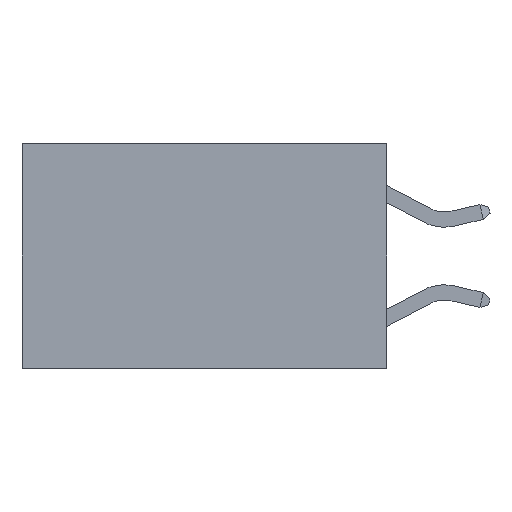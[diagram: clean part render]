
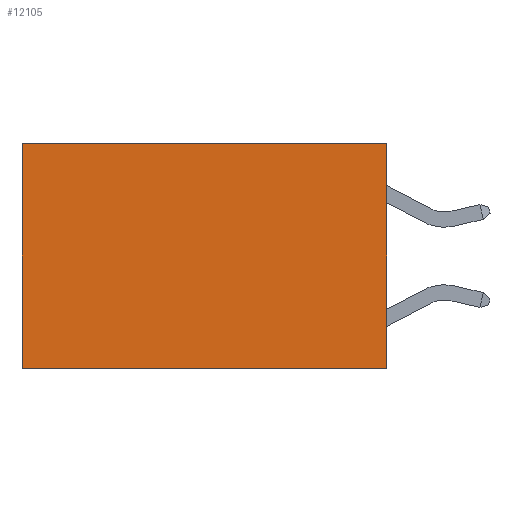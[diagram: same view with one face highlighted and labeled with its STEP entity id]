
A CAD part, left-side view. The second image highlights one B-rep face of the part: STEP entity #12105.
In plain terms, the highlighted planar face has unit normal (-1, 0, 0).
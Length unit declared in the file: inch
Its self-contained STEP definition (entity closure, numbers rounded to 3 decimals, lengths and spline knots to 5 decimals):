
#593 = DIRECTION ( 'NONE',  ( 0., 1., 0. ) ) ;
#1850 = VERTEX_POINT ( 'NONE', #5355 ) ;
#2541 = DIRECTION ( 'NONE',  ( 0., 1., 0. ) ) ;
#3790 = VECTOR ( 'NONE', #593, 39.37008 ) ;
#4301 = CARTESIAN_POINT ( 'NONE',  ( 0.2625, 0., 0. ) ) ;
#4383 = LINE ( 'NONE', #5997, #3790 ) ;
#4386 = DIRECTION ( 'NONE',  ( 0., 0., -1. ) ) ;
#4781 = AXIS2_PLACEMENT_3D ( 'NONE', #4301, #15117, #4386 ) ;
#5355 = CARTESIAN_POINT ( 'NONE',  ( 0.2625, 0., 0. ) ) ;
#5995 = VECTOR ( 'NONE', #2541, 39.37008 ) ;
#5997 = CARTESIAN_POINT ( 'NONE',  ( 0.2625, 0., -0.37 ) ) ;
#6035 = DIRECTION ( 'NONE',  ( 0., 0., -1. ) ) ;
#6043 = VECTOR ( 'NONE', #6035, 39.37008 ) ;
#6284 = LINE ( 'NONE', #15484, #19985 ) ;
#7701 = EDGE_CURVE ( 'NONE', #8911, #21904, #4383, .T. ) ;
#7807 = CARTESIAN_POINT ( 'NONE',  ( 0.2625, 0.6, 0. ) ) ;
#8381 = CARTESIAN_POINT ( 'NONE',  ( 0.2625, 0.6, 0. ) ) ;
#8502 = DIRECTION ( 'NONE',  ( 0., 0., -1. ) ) ;
#8504 = EDGE_CURVE ( 'NONE', #11580, #21904, #10812, .T. ) ;
#8738 = ORIENTED_EDGE ( 'NONE', *, *, #7701, .F. ) ;
#8911 = VERTEX_POINT ( 'NONE', #12494 ) ;
#10050 = EDGE_LOOP ( 'NONE', ( #18749, #8738, #15216, #20213 ) ) ;
#10812 = LINE ( 'NONE', #7807, #6043 ) ;
#11580 = VERTEX_POINT ( 'NONE', #8381 ) ;
#12105 = ADVANCED_FACE ( 'NONE', ( #21816 ), #22216, .F. ) ;
#12494 = CARTESIAN_POINT ( 'NONE',  ( 0.2625, 0., -0.37 ) ) ;
#13863 = CARTESIAN_POINT ( 'NONE',  ( 0.2625, 0.6, -0.37 ) ) ;
#15117 = DIRECTION ( 'NONE',  ( 1., 0., 0. ) ) ;
#15216 = ORIENTED_EDGE ( 'NONE', *, *, #19583, .F. ) ;
#15484 = CARTESIAN_POINT ( 'NONE',  ( 0.2625, 0., 0. ) ) ;
#18749 = ORIENTED_EDGE ( 'NONE', *, *, #8504, .T. ) ;
#19583 = EDGE_CURVE ( 'NONE', #1850, #8911, #6284, .T. ) ;
#19985 = VECTOR ( 'NONE', #8502, 39.37008 ) ;
#20213 = ORIENTED_EDGE ( 'NONE', *, *, #20654, .T. ) ;
#20262 = LINE ( 'NONE', #20440, #5995 ) ;
#20440 = CARTESIAN_POINT ( 'NONE',  ( 0.2625, 0., 0. ) ) ;
#20654 = EDGE_CURVE ( 'NONE', #1850, #11580, #20262, .T. ) ;
#21816 = FACE_OUTER_BOUND ( 'NONE', #10050, .T. ) ;
#21904 = VERTEX_POINT ( 'NONE', #13863 ) ;
#22216 = PLANE ( 'NONE',  #4781 ) ;
